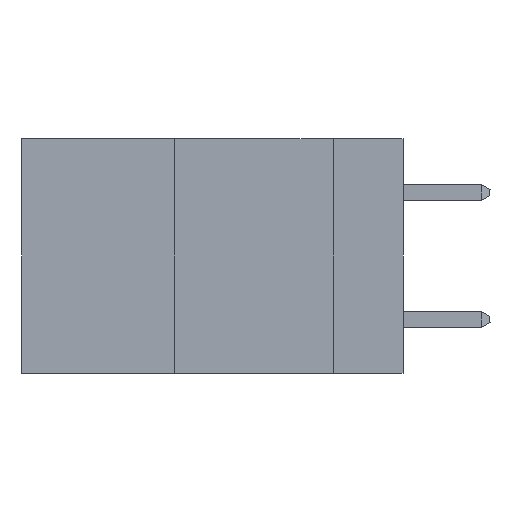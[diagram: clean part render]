
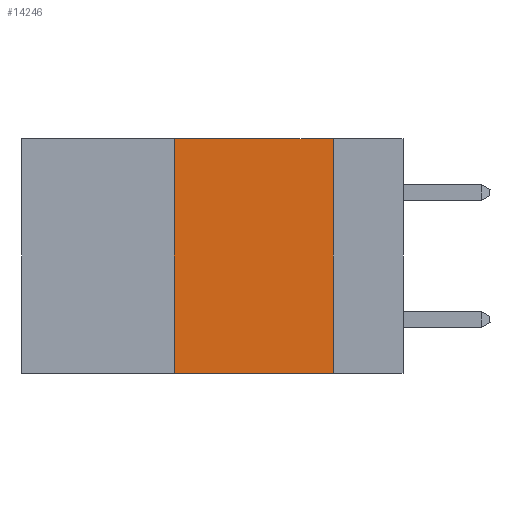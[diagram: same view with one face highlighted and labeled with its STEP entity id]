
A CAD part, left-side view. The second image highlights one B-rep face of the part: STEP entity #14246.
In plain terms, the highlighted planar face has unit normal (-1, 0, 0).
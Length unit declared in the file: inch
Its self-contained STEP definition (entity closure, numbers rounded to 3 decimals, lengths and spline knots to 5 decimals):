
#1356 = CARTESIAN_POINT ( 'NONE',  ( 0., 0.36, 0. ) ) ;
#1416 = CARTESIAN_POINT ( 'NONE',  ( 0., 0.11, 0. ) ) ;
#2552 = LINE ( 'NONE', #25989, #25801 ) ;
#3400 = EDGE_CURVE ( 'NONE', #6932, #19054, #22544, .T. ) ;
#6932 = VERTEX_POINT ( 'NONE', #13009 ) ;
#7910 = VECTOR ( 'NONE', #8154, 39.37008 ) ;
#8154 = DIRECTION ( 'NONE',  ( 0., 0., 1. ) ) ;
#8795 = FACE_OUTER_BOUND ( 'NONE', #17728, .T. ) ;
#8989 = ORIENTED_EDGE ( 'NONE', *, *, #30140, .F. ) ;
#10074 = EDGE_CURVE ( 'NONE', #24901, #19054, #2552, .T. ) ;
#11176 = ORIENTED_EDGE ( 'NONE', *, *, #27988, .F. ) ;
#11455 = LINE ( 'NONE', #28988, #7910 ) ;
#13009 = CARTESIAN_POINT ( 'NONE',  ( 0., 0.36, -0.37 ) ) ;
#13090 = PLANE ( 'NONE',  #31568 ) ;
#13346 = VECTOR ( 'NONE', #21717, 39.37008 ) ;
#14246 = ADVANCED_FACE ( 'NONE', ( #8795 ), #13090, .F. ) ;
#16124 = LINE ( 'NONE', #29544, #13346 ) ;
#17172 = ORIENTED_EDGE ( 'NONE', *, *, #3400, .T. ) ;
#17728 = EDGE_LOOP ( 'NONE', ( #28155, #8989, #11176, #17172 ) ) ;
#17761 = VECTOR ( 'NONE', #23034, 39.37008 ) ;
#19054 = VERTEX_POINT ( 'NONE', #19978 ) ;
#19978 = CARTESIAN_POINT ( 'NONE',  ( 0., 0.11, -0.37 ) ) ;
#20471 = CARTESIAN_POINT ( 'NONE',  ( 0., 0.6, -0.37 ) ) ;
#21717 = DIRECTION ( 'NONE',  ( 0., -1., 0. ) ) ;
#21763 = DIRECTION ( 'NONE',  ( 1., 0., 0. ) ) ;
#22544 = LINE ( 'NONE', #20471, #17761 ) ;
#23034 = DIRECTION ( 'NONE',  ( 0., -1., 0. ) ) ;
#24236 = DIRECTION ( 'NONE',  ( 0., 0., -1. ) ) ;
#24901 = VERTEX_POINT ( 'NONE', #1416 ) ;
#25801 = VECTOR ( 'NONE', #26621, 39.37008 ) ;
#25989 = CARTESIAN_POINT ( 'NONE',  ( 0., 0.11, 0. ) ) ;
#26621 = DIRECTION ( 'NONE',  ( 0., 0., -1. ) ) ;
#27988 = EDGE_CURVE ( 'NONE', #6932, #32585, #11455, .T. ) ;
#28155 = ORIENTED_EDGE ( 'NONE', *, *, #10074, .F. ) ;
#28594 = CARTESIAN_POINT ( 'NONE',  ( 0., 0.6, 0. ) ) ;
#28988 = CARTESIAN_POINT ( 'NONE',  ( 0., 0.36, 0. ) ) ;
#29544 = CARTESIAN_POINT ( 'NONE',  ( 0., 0.6, 0. ) ) ;
#30140 = EDGE_CURVE ( 'NONE', #32585, #24901, #16124, .T. ) ;
#31568 = AXIS2_PLACEMENT_3D ( 'NONE', #28594, #21763, #24236 ) ;
#32585 = VERTEX_POINT ( 'NONE', #1356 ) ;
